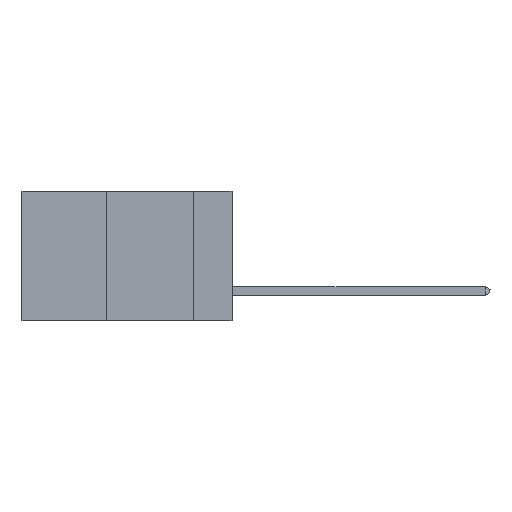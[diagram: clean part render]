
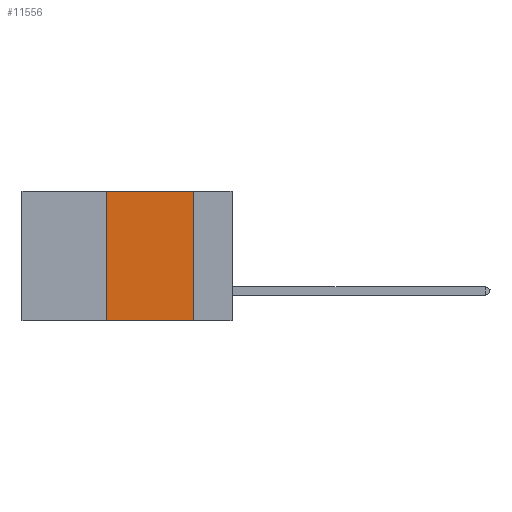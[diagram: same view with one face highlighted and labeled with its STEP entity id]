
A CAD part, left-side view. The second image highlights one B-rep face of the part: STEP entity #11556.
In plain terms, the highlighted planar face has unit normal (-1, 0, 0).
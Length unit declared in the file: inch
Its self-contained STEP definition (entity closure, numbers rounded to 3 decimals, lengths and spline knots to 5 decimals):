
#3973 = EDGE_CURVE ( 'NONE', #37497, #19559, #41538, .T. ) ;
#4755 = LINE ( 'NONE', #30591, #36931 ) ;
#6704 = CARTESIAN_POINT ( 'NONE',  ( 0., 0.6, 0. ) ) ;
#8103 = VECTOR ( 'NONE', #40323, 39.37008 ) ;
#8602 = EDGE_CURVE ( 'NONE', #19559, #45241, #19034, .T. ) ;
#9314 = LINE ( 'NONE', #40012, #8103 ) ;
#11520 = ORIENTED_EDGE ( 'NONE', *, *, #8602, .F. ) ;
#11556 = ADVANCED_FACE ( 'NONE', ( #23353 ), #20856, .F. ) ;
#12749 = CARTESIAN_POINT ( 'NONE',  ( 0., 0.11, 0. ) ) ;
#13433 = EDGE_CURVE ( 'NONE', #28743, #45241, #9314, .T. ) ;
#14247 = DIRECTION ( 'NONE',  ( 0., -1., 0. ) ) ;
#15439 = CARTESIAN_POINT ( 'NONE',  ( 0., 0.36, 0. ) ) ;
#17282 = CARTESIAN_POINT ( 'NONE',  ( 0., 0.11, 0. ) ) ;
#19034 = LINE ( 'NONE', #17282, #47628 ) ;
#19220 = CARTESIAN_POINT ( 'NONE',  ( 0., 0.11, -0.37 ) ) ;
#19559 = VERTEX_POINT ( 'NONE', #12749 ) ;
#20329 = EDGE_CURVE ( 'NONE', #28743, #37497, #4755, .T. ) ;
#20491 = EDGE_LOOP ( 'NONE', ( #11520, #47796, #36344, #45833 ) ) ;
#20856 = PLANE ( 'NONE',  #44784 ) ;
#21020 = DIRECTION ( 'NONE',  ( 0., 0., -1. ) ) ;
#23353 = FACE_OUTER_BOUND ( 'NONE', #20491, .T. ) ;
#28743 = VERTEX_POINT ( 'NONE', #35457 ) ;
#30591 = CARTESIAN_POINT ( 'NONE',  ( 0., 0.36, 0. ) ) ;
#35457 = CARTESIAN_POINT ( 'NONE',  ( 0., 0.36, -0.37 ) ) ;
#36344 = ORIENTED_EDGE ( 'NONE', *, *, #20329, .F. ) ;
#36931 = VECTOR ( 'NONE', #41847, 39.37008 ) ;
#37497 = VERTEX_POINT ( 'NONE', #15439 ) ;
#39814 = DIRECTION ( 'NONE',  ( 1., 0., 0. ) ) ;
#40012 = CARTESIAN_POINT ( 'NONE',  ( 0., 0.6, -0.37 ) ) ;
#40185 = CARTESIAN_POINT ( 'NONE',  ( 0., 0.6, 0. ) ) ;
#40323 = DIRECTION ( 'NONE',  ( 0., -1., 0. ) ) ;
#41538 = LINE ( 'NONE', #40185, #42701 ) ;
#41847 = DIRECTION ( 'NONE',  ( 0., 0., 1. ) ) ;
#42701 = VECTOR ( 'NONE', #14247, 39.37008 ) ;
#43817 = DIRECTION ( 'NONE',  ( 0., 0., -1. ) ) ;
#44784 = AXIS2_PLACEMENT_3D ( 'NONE', #6704, #39814, #43817 ) ;
#45241 = VERTEX_POINT ( 'NONE', #19220 ) ;
#45833 = ORIENTED_EDGE ( 'NONE', *, *, #13433, .T. ) ;
#47628 = VECTOR ( 'NONE', #21020, 39.37008 ) ;
#47796 = ORIENTED_EDGE ( 'NONE', *, *, #3973, .F. ) ;
